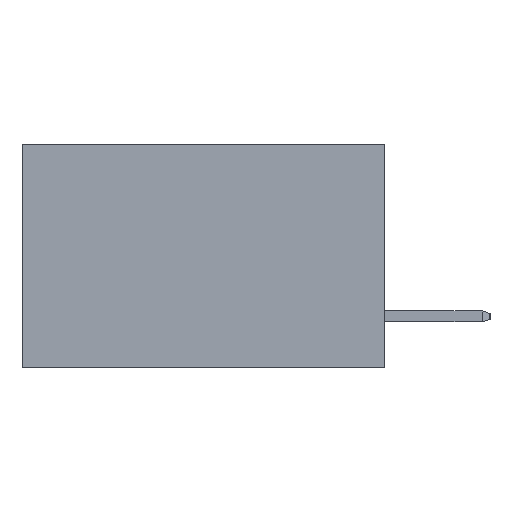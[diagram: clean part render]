
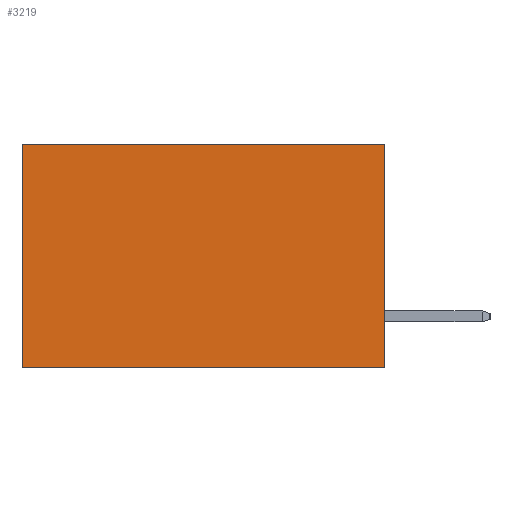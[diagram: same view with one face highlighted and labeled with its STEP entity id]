
A CAD part, left-side view. The second image highlights one B-rep face of the part: STEP entity #3219.
In plain terms, the highlighted planar face has unit normal (-1, 0, 0).
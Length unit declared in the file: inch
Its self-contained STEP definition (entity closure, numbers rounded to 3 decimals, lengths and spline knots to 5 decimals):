
#584 = VECTOR ( 'NONE', #2301, 39.37008 ) ;
#817 = DIRECTION ( 'NONE',  ( 1., 0., 0. ) ) ;
#1028 = CARTESIAN_POINT ( 'NONE',  ( 0.298, 0., -0.37 ) ) ;
#1442 = EDGE_CURVE ( 'NONE', #1696, #6194, #12612, .T. ) ;
#1696 = VERTEX_POINT ( 'NONE', #8579 ) ;
#2301 = DIRECTION ( 'NONE',  ( 0., 0., -1. ) ) ;
#2467 = DIRECTION ( 'NONE',  ( 0., 1., 0. ) ) ;
#3219 = ADVANCED_FACE ( 'NONE', ( #18348 ), #3566, .F. ) ;
#3296 = VERTEX_POINT ( 'NONE', #12822 ) ;
#3566 = PLANE ( 'NONE',  #11833 ) ;
#3573 = CARTESIAN_POINT ( 'NONE',  ( 0.298, 0., 0. ) ) ;
#3694 = LINE ( 'NONE', #13049, #14815 ) ;
#4529 = ORIENTED_EDGE ( 'NONE', *, *, #6190, .F. ) ;
#5963 = EDGE_LOOP ( 'NONE', ( #9441, #4529, #14232, #14277 ) ) ;
#6109 = CARTESIAN_POINT ( 'NONE',  ( 0.298, 0., 0. ) ) ;
#6190 = EDGE_CURVE ( 'NONE', #6194, #10334, #8404, .T. ) ;
#6194 = VERTEX_POINT ( 'NONE', #1028 ) ;
#7375 = VECTOR ( 'NONE', #2467, 39.37008 ) ;
#7864 = EDGE_CURVE ( 'NONE', #1696, #3296, #11182, .T. ) ;
#8404 = LINE ( 'NONE', #14584, #11772 ) ;
#8579 = CARTESIAN_POINT ( 'NONE',  ( 0.298, 0., 0. ) ) ;
#8921 = CARTESIAN_POINT ( 'NONE',  ( 0.298, 0.6, -0.37 ) ) ;
#9441 = ORIENTED_EDGE ( 'NONE', *, *, #18221, .T. ) ;
#10334 = VERTEX_POINT ( 'NONE', #8921 ) ;
#11182 = LINE ( 'NONE', #6109, #7375 ) ;
#11772 = VECTOR ( 'NONE', #13324, 39.37008 ) ;
#11833 = AXIS2_PLACEMENT_3D ( 'NONE', #3573, #817, #14172 ) ;
#12612 = LINE ( 'NONE', #18375, #584 ) ;
#12822 = CARTESIAN_POINT ( 'NONE',  ( 0.298, 0.6, 0. ) ) ;
#13049 = CARTESIAN_POINT ( 'NONE',  ( 0.298, 0.6, 0. ) ) ;
#13324 = DIRECTION ( 'NONE',  ( 0., 1., 0. ) ) ;
#14172 = DIRECTION ( 'NONE',  ( 0., 0., -1. ) ) ;
#14232 = ORIENTED_EDGE ( 'NONE', *, *, #1442, .F. ) ;
#14277 = ORIENTED_EDGE ( 'NONE', *, *, #7864, .T. ) ;
#14524 = DIRECTION ( 'NONE',  ( 0., 0., -1. ) ) ;
#14584 = CARTESIAN_POINT ( 'NONE',  ( 0.298, 0., -0.37 ) ) ;
#14815 = VECTOR ( 'NONE', #14524, 39.37008 ) ;
#18221 = EDGE_CURVE ( 'NONE', #3296, #10334, #3694, .T. ) ;
#18348 = FACE_OUTER_BOUND ( 'NONE', #5963, .T. ) ;
#18375 = CARTESIAN_POINT ( 'NONE',  ( 0.298, 0., 0. ) ) ;
